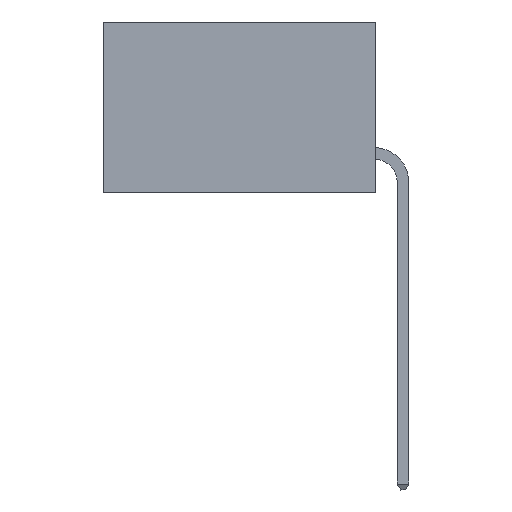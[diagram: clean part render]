
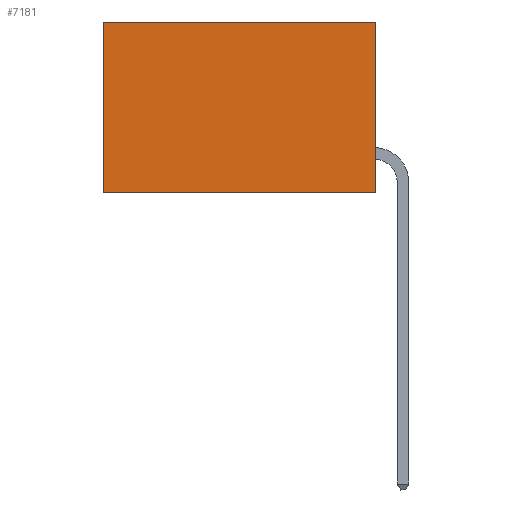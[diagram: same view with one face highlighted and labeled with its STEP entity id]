
A CAD part, left-side view. The second image highlights one B-rep face of the part: STEP entity #7181.
In plain terms, the highlighted planar face has unit normal (-1, 0, 0).
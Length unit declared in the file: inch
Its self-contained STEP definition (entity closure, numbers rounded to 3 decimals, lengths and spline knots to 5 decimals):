
#25 = VECTOR ( 'NONE', #6940, 39.37008 ) ;
#37 = LINE ( 'NONE', #8022, #8416 ) ;
#93 = VERTEX_POINT ( 'NONE', #2406 ) ;
#116 = VECTOR ( 'NONE', #7929, 39.37008 ) ;
#555 = CARTESIAN_POINT ( 'NONE',  ( 0.277, 0., -0.37 ) ) ;
#882 = ORIENTED_EDGE ( 'NONE', *, *, #4148, .T. ) ;
#896 = EDGE_CURVE ( 'NONE', #6330, #2195, #37, .T. ) ;
#988 = ORIENTED_EDGE ( 'NONE', *, *, #3012, .F. ) ;
#1102 = EDGE_CURVE ( 'NONE', #6330, #10147, #2540, .T. ) ;
#1258 = ORIENTED_EDGE ( 'NONE', *, *, #1102, .F. ) ;
#1295 = ORIENTED_EDGE ( 'NONE', *, *, #896, .T. ) ;
#1315 = FACE_OUTER_BOUND ( 'NONE', #9011, .T. ) ;
#1608 = AXIS2_PLACEMENT_3D ( 'NONE', #8449, #8241, #7106 ) ;
#2195 = VERTEX_POINT ( 'NONE', #2895 ) ;
#2392 = VECTOR ( 'NONE', #3215, 39.37008 ) ;
#2406 = CARTESIAN_POINT ( 'NONE',  ( 0.277, 0.59, -0.37 ) ) ;
#2540 = LINE ( 'NONE', #6903, #25 ) ;
#2895 = CARTESIAN_POINT ( 'NONE',  ( 0.277, 0.59, 0. ) ) ;
#3012 = EDGE_CURVE ( 'NONE', #10147, #93, #4484, .T. ) ;
#3215 = DIRECTION ( 'NONE',  ( 0., 1., 0. ) ) ;
#4148 = EDGE_CURVE ( 'NONE', #2195, #93, #4925, .T. ) ;
#4484 = LINE ( 'NONE', #5144, #2392 ) ;
#4925 = LINE ( 'NONE', #5242, #116 ) ;
#5144 = CARTESIAN_POINT ( 'NONE',  ( 0.277, 0., -0.37 ) ) ;
#5242 = CARTESIAN_POINT ( 'NONE',  ( 0.277, 0.59, -0.37 ) ) ;
#5287 = DIRECTION ( 'NONE',  ( 0., 1., 0. ) ) ;
#6330 = VERTEX_POINT ( 'NONE', #8254 ) ;
#6903 = CARTESIAN_POINT ( 'NONE',  ( 0.277, 0., -0.37 ) ) ;
#6940 = DIRECTION ( 'NONE',  ( 0., 0., -1. ) ) ;
#7106 = DIRECTION ( 'NONE',  ( 0., 0., -1. ) ) ;
#7181 = ADVANCED_FACE ( 'NONE', ( #1315 ), #8297, .F. ) ;
#7929 = DIRECTION ( 'NONE',  ( 0., 0., -1. ) ) ;
#8022 = CARTESIAN_POINT ( 'NONE',  ( 0.277, 0., 0. ) ) ;
#8241 = DIRECTION ( 'NONE',  ( 1., 0., 0. ) ) ;
#8254 = CARTESIAN_POINT ( 'NONE',  ( 0.277, 0., 0. ) ) ;
#8297 = PLANE ( 'NONE',  #1608 ) ;
#8416 = VECTOR ( 'NONE', #5287, 39.37008 ) ;
#8449 = CARTESIAN_POINT ( 'NONE',  ( 0.277, 0., -0.37 ) ) ;
#9011 = EDGE_LOOP ( 'NONE', ( #882, #988, #1258, #1295 ) ) ;
#10147 = VERTEX_POINT ( 'NONE', #555 ) ;
